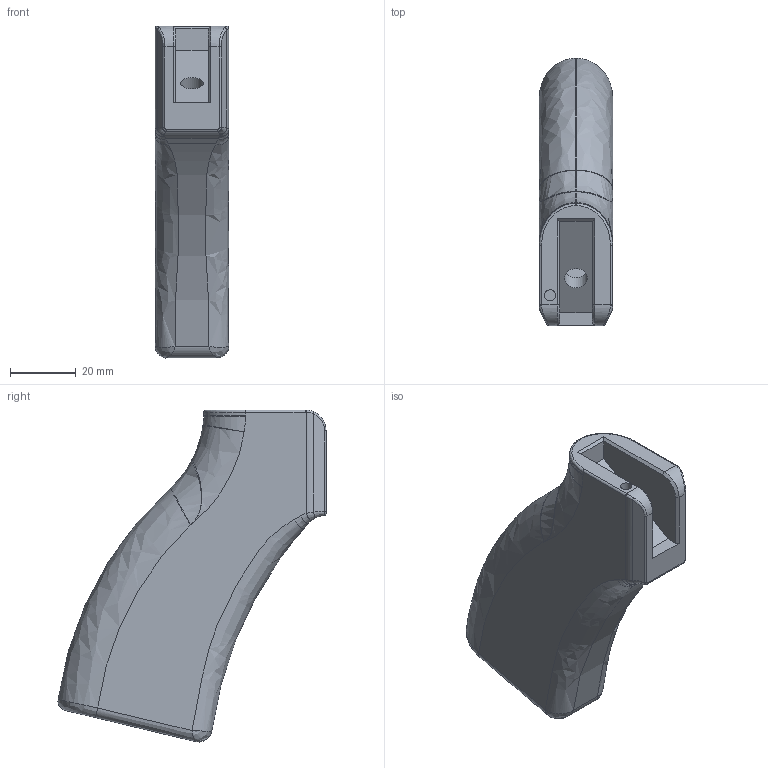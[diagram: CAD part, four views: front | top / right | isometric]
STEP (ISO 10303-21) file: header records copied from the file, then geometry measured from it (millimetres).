
FILE_DESCRIPTION(/* description */ (''),/* implementation_level */ '2;1');
FILE_NAME(/* name */ 'CQ Grip.step',/* time_stamp */ '2021-04-13T12:09:54-04:00',/* author */ (''),/* organization */ (''),/* preprocessor_version */ 'ST-DEVELOPER v18.1',/* originating_system */ 'Autodesk Translation Framework v10.6.0.1341',/* authorisation */ '');
FILE_SCHEMA (('AUTOMOTIVE_DESIGN { 1 0 10303 214 3 1 1 }'));
Length unit declared in the file: millimetre
Products named in the file (1): CQ Grip
Bounding box: 22.33 x 81.51 x 100.96 mm (x, y, z)
Volume: 53192 mm3; surface area: 22447.5 mm2
Topology: 1 solids, 1 shells, 142 faces, 327 edges, 173 vertices
Faces by surface type: bspline 54, cylinder 42, plane 31, torus 8, cone 5, sphere 2
Full cylindrical faces by diameter (mm): 3.4 x1, 6.8 x1
Entity records: 6319 total; most frequent: CARTESIAN_POINT 3482, ORIENTED_EDGE 622, DIRECTION 501, EDGE_CURVE 311, AXIS2_PLACEMENT_3D 190, VERTEX_POINT 173, EDGE_LOOP 146, FACE_OUTER_BOUND 142
